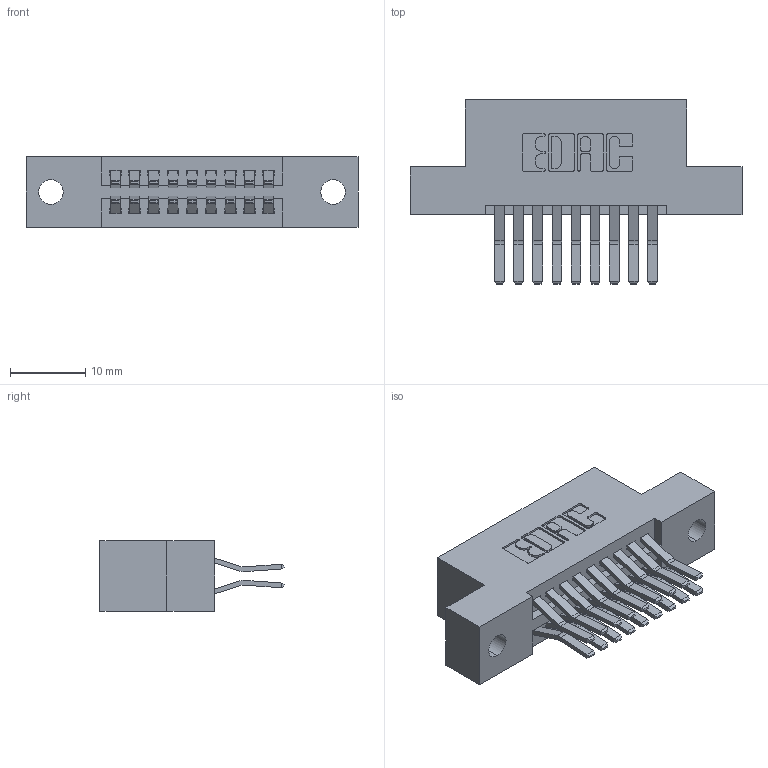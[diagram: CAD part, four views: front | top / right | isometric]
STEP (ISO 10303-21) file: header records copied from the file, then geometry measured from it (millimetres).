
FILE_DESCRIPTION (( 'STEP AP203' ), '1' );
FILE_NAME ('395-018-560-202.STEP', '2018-11-07T04:43:54', ( '' ), ( '' ), 'SwSTEP 2.0', 'SolidWorks 2016', '' );
FILE_SCHEMA (( 'CONFIG_CONTROL_DESIGN' ));
Length unit declared in the file: inch
Products named in the file (3): 345-292-001_560 Tail; 395-018-560-202; 345 Part_Flush Mounting Lugs - 0.128 Dia
Assembly tree (19 placements, depth 2):
  395-018-560-202
    345 Part_Flush Mounting Lugs - 0.128 Dia
    345-292-001_560 Tail  x18
Bounding box: 44.07 x 24.45 x 9.4 mm (x, y, z)
Volume: 4055.9 mm3; surface area: 5386.9 mm2
Topology: 19 solids, 19 shells, 1062 faces, 3131 edges, 2062 vertices
Faces by surface type: plane 674, cylinder 388
Entity records: 11595 total; most frequent: CARTESIAN_POINT 1976, ORIENTED_EDGE 1910, DIRECTION 1787, EDGE_CURVE 955, VECTOR 783, LINE 783, VERTEX_POINT 634, AXIS2_PLACEMENT_3D 502
